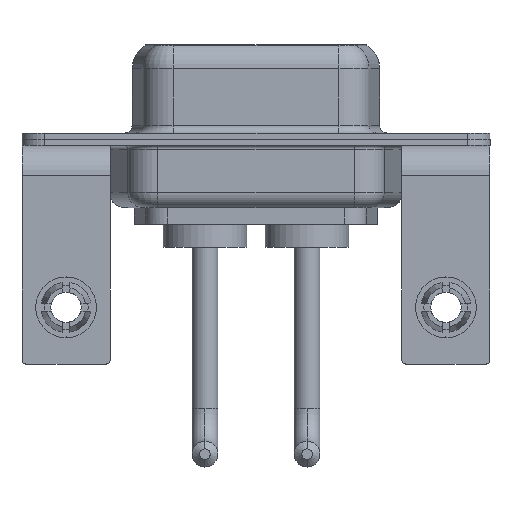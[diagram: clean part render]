
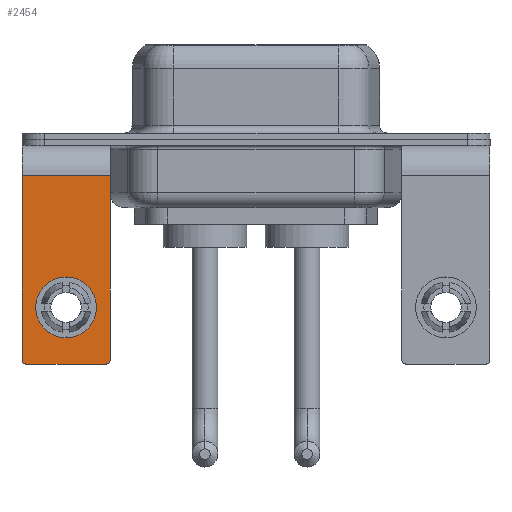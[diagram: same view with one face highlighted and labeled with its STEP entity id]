
A CAD part, front view. The second image highlights one B-rep face of the part: STEP entity #2454.
In plain terms, the highlighted planar face has unit normal (0, -1, 0).
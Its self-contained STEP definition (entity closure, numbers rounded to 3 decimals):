
#833 = EDGE_CURVE ( 'NONE', #7358, #12690, #5776, .T. ) ;
#1146 = LINE ( 'NONE', #9906, #10270 ) ;
#1865 = DIRECTION ( 'NONE',  ( 0., 1., 0. ) ) ;
#1950 = DIRECTION ( 'NONE',  ( 0., -1., 0. ) ) ;
#2335 = LINE ( 'NONE', #8942, #3324 ) ;
#2401 = CARTESIAN_POINT ( 'NONE',  ( -2.65, -6.25, -14.55 ) ) ;
#2454 = ADVANCED_FACE ( 'NONE', ( #13420, #11205 ), #3338, .F. ) ;
#2587 = AXIS2_PLACEMENT_3D ( 'NONE', #10997, #1950, #11890 ) ;
#2786 = ORIENTED_EDGE ( 'NONE', *, *, #4900, .T. ) ;
#2930 = CARTESIAN_POINT ( 'NONE',  ( 0., -6.25, -9.07 ) ) ;
#3182 = VERTEX_POINT ( 'NONE', #2930 ) ;
#3324 = VECTOR ( 'NONE', #10271, 1000. ) ;
#3338 = PLANE ( 'NONE',  #3518 ) ;
#3420 = DIRECTION ( 'NONE',  ( -1., 0., 0. ) ) ;
#3518 = AXIS2_PLACEMENT_3D ( 'NONE', #7822, #4208, #11136 ) ;
#3540 = AXIS2_PLACEMENT_3D ( 'NONE', #10055, #7779, #6404 ) ;
#3620 = EDGE_CURVE ( 'NONE', #7358, #12888, #2335, .T. ) ;
#3908 = DIRECTION ( 'NONE',  ( 0., 0., 1. ) ) ;
#4077 = ORIENTED_EDGE ( 'NONE', *, *, #833, .F. ) ;
#4208 = DIRECTION ( 'NONE',  ( 0., 1., 0. ) ) ;
#4324 = LINE ( 'NONE', #7865, #7561 ) ;
#4344 = EDGE_CURVE ( 'NONE', #12362, #3182, #9226, .T. ) ;
#4900 = EDGE_CURVE ( 'NONE', #12888, #10272, #4324, .T. ) ;
#5052 = CARTESIAN_POINT ( 'NONE',  ( -2.9, -6.25, -14.55 ) ) ;
#5326 = CARTESIAN_POINT ( 'NONE',  ( 0., -6.25, -11.07 ) ) ;
#5374 = CARTESIAN_POINT ( 'NONE',  ( 2.9, -6.25, -14.55 ) ) ;
#5776 = LINE ( 'NONE', #11590, #5986 ) ;
#5942 = ORIENTED_EDGE ( 'NONE', *, *, #4344, .T. ) ;
#5986 = VECTOR ( 'NONE', #11517, 1000. ) ;
#6404 = DIRECTION ( 'NONE',  ( 0., 0., 1. ) ) ;
#6590 = VERTEX_POINT ( 'NONE', #8082 ) ;
#7133 = AXIS2_PLACEMENT_3D ( 'NONE', #5326, #1865, #14385 ) ;
#7260 = EDGE_CURVE ( 'NONE', #8190, #6590, #1146, .T. ) ;
#7358 = VERTEX_POINT ( 'NONE', #11010 ) ;
#7512 = EDGE_CURVE ( 'NONE', #10272, #6590, #12879, .T. ) ;
#7561 = VECTOR ( 'NONE', #13530, 1000. ) ;
#7779 = DIRECTION ( 'NONE',  ( 0., 1., 0. ) ) ;
#7822 = CARTESIAN_POINT ( 'NONE',  ( 2.9, -6.25, -2.4 ) ) ;
#7865 = CARTESIAN_POINT ( 'NONE',  ( -2.9, -6.25, -2.4 ) ) ;
#8082 = CARTESIAN_POINT ( 'NONE',  ( -2.65, -6.25, -14.8 ) ) ;
#8190 = VERTEX_POINT ( 'NONE', #12071 ) ;
#8529 = ORIENTED_EDGE ( 'NONE', *, *, #7260, .F. ) ;
#8656 = ORIENTED_EDGE ( 'NONE', *, *, #13241, .T. ) ;
#8674 = ORIENTED_EDGE ( 'NONE', *, *, #3620, .T. ) ;
#8942 = CARTESIAN_POINT ( 'NONE',  ( 2.9, -6.25, -2.4 ) ) ;
#9226 = CIRCLE ( 'NONE', #7133, 2. ) ;
#9382 = CIRCLE ( 'NONE', #2587, 0.25 ) ;
#9741 = CARTESIAN_POINT ( 'NONE',  ( 0., -6.25, -13.07 ) ) ;
#9906 = CARTESIAN_POINT ( 'NONE',  ( 2.9, -6.25, -14.8 ) ) ;
#10055 = CARTESIAN_POINT ( 'NONE',  ( 0., -6.25, -11.07 ) ) ;
#10270 = VECTOR ( 'NONE', #3420, 1000. ) ;
#10271 = DIRECTION ( 'NONE',  ( -1., 0., 0. ) ) ;
#10272 = VERTEX_POINT ( 'NONE', #5052 ) ;
#10467 = ORIENTED_EDGE ( 'NONE', *, *, #12268, .T. ) ;
#10997 = CARTESIAN_POINT ( 'NONE',  ( 2.65, -6.25, -14.55 ) ) ;
#11010 = CARTESIAN_POINT ( 'NONE',  ( 2.9, -6.25, -2.4 ) ) ;
#11136 = DIRECTION ( 'NONE',  ( 0., 0., 1. ) ) ;
#11205 = FACE_OUTER_BOUND ( 'NONE', #14502, .T. ) ;
#11452 = AXIS2_PLACEMENT_3D ( 'NONE', #2401, #11721, #3908 ) ;
#11470 = CARTESIAN_POINT ( 'NONE',  ( -2.9, -6.25, -2.4 ) ) ;
#11517 = DIRECTION ( 'NONE',  ( 0., 0., -1. ) ) ;
#11590 = CARTESIAN_POINT ( 'NONE',  ( 2.9, -6.25, -2.4 ) ) ;
#11721 = DIRECTION ( 'NONE',  ( 0., -1., 0. ) ) ;
#11890 = DIRECTION ( 'NONE',  ( 0., 0., 1. ) ) ;
#12007 = ORIENTED_EDGE ( 'NONE', *, *, #7512, .T. ) ;
#12071 = CARTESIAN_POINT ( 'NONE',  ( 2.65, -6.25, -14.8 ) ) ;
#12247 = CIRCLE ( 'NONE', #3540, 2. ) ;
#12268 = EDGE_CURVE ( 'NONE', #8190, #12690, #9382, .T. ) ;
#12362 = VERTEX_POINT ( 'NONE', #9741 ) ;
#12690 = VERTEX_POINT ( 'NONE', #5374 ) ;
#12879 = CIRCLE ( 'NONE', #11452, 0.25 ) ;
#12888 = VERTEX_POINT ( 'NONE', #11470 ) ;
#13241 = EDGE_CURVE ( 'NONE', #3182, #12362, #12247, .T. ) ;
#13412 = EDGE_LOOP ( 'NONE', ( #5942, #8656 ) ) ;
#13420 = FACE_BOUND ( 'NONE', #13412, .T. ) ;
#13530 = DIRECTION ( 'NONE',  ( 0., 0., -1. ) ) ;
#14385 = DIRECTION ( 'NONE',  ( 0., 0., 1. ) ) ;
#14502 = EDGE_LOOP ( 'NONE', ( #2786, #12007, #8529, #10467, #4077, #8674 ) ) ;
